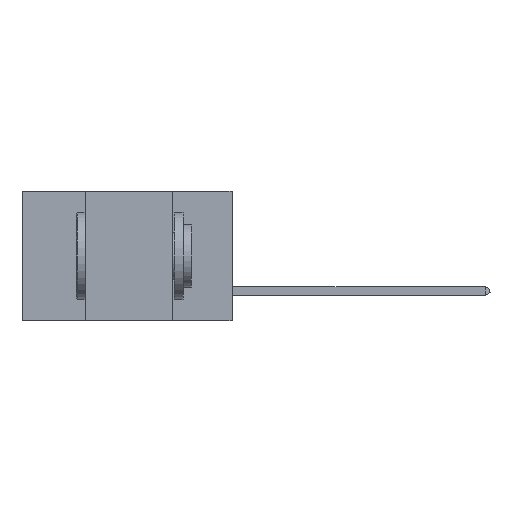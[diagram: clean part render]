
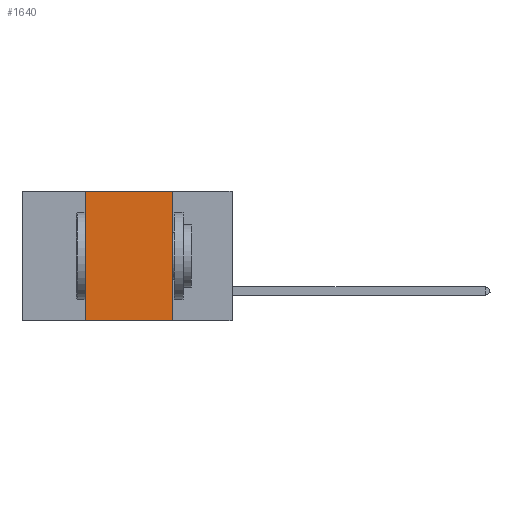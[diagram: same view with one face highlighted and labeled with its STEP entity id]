
A CAD part, left-side view. The second image highlights one B-rep face of the part: STEP entity #1640.
In plain terms, the highlighted planar face has unit normal (-1, 0, 0).
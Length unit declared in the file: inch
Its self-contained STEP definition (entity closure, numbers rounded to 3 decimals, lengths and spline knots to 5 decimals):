
#347 = VERTEX_POINT ( 'NONE', #4210 ) ;
#1179 = DIRECTION ( 'NONE',  ( 0., 0., -1. ) ) ;
#1640 = ADVANCED_FACE ( 'NONE', ( #12622 ), #4724, .F. ) ;
#1885 = CARTESIAN_POINT ( 'NONE',  ( 0., 0.17, 0. ) ) ;
#2037 = VECTOR ( 'NONE', #13070, 39.37008 ) ;
#3229 = VERTEX_POINT ( 'NONE', #1885 ) ;
#3292 = LINE ( 'NONE', #4136, #15643 ) ;
#4108 = EDGE_CURVE ( 'NONE', #347, #5937, #15225, .T. ) ;
#4136 = CARTESIAN_POINT ( 'NONE',  ( 0., 0.6, 0. ) ) ;
#4210 = CARTESIAN_POINT ( 'NONE',  ( 0., 0.42, -0.37 ) ) ;
#4724 = PLANE ( 'NONE',  #19978 ) ;
#4858 = DIRECTION ( 'NONE',  ( 1., 0., 0. ) ) ;
#4985 = LINE ( 'NONE', #20111, #16313 ) ;
#5413 = CARTESIAN_POINT ( 'NONE',  ( 0., 0.42, 0. ) ) ;
#5586 = VECTOR ( 'NONE', #18313, 39.37008 ) ;
#5937 = VERTEX_POINT ( 'NONE', #5413 ) ;
#6559 = ORIENTED_EDGE ( 'NONE', *, *, #7657, .F. ) ;
#7657 = EDGE_CURVE ( 'NONE', #5937, #3229, #3292, .T. ) ;
#7840 = CARTESIAN_POINT ( 'NONE',  ( 0., 0.6, 0. ) ) ;
#8674 = EDGE_CURVE ( 'NONE', #3229, #16984, #4985, .T. ) ;
#10246 = DIRECTION ( 'NONE',  ( 0., -1., 0. ) ) ;
#10285 = CARTESIAN_POINT ( 'NONE',  ( 0., 0.17, -0.37 ) ) ;
#10516 = ORIENTED_EDGE ( 'NONE', *, *, #18574, .T. ) ;
#12622 = FACE_OUTER_BOUND ( 'NONE', #14858, .T. ) ;
#13070 = DIRECTION ( 'NONE',  ( 0., -1., 0. ) ) ;
#14394 = DIRECTION ( 'NONE',  ( 0., 0., -1. ) ) ;
#14858 = EDGE_LOOP ( 'NONE', ( #19906, #6559, #18396, #10516 ) ) ;
#14912 = CARTESIAN_POINT ( 'NONE',  ( 0., 0.6, -0.37 ) ) ;
#15225 = LINE ( 'NONE', #16686, #5586 ) ;
#15643 = VECTOR ( 'NONE', #10246, 39.37008 ) ;
#16313 = VECTOR ( 'NONE', #1179, 39.37008 ) ;
#16686 = CARTESIAN_POINT ( 'NONE',  ( 0., 0.42, 0. ) ) ;
#16836 = LINE ( 'NONE', #14912, #2037 ) ;
#16984 = VERTEX_POINT ( 'NONE', #10285 ) ;
#18313 = DIRECTION ( 'NONE',  ( 0., 0., 1. ) ) ;
#18396 = ORIENTED_EDGE ( 'NONE', *, *, #4108, .F. ) ;
#18574 = EDGE_CURVE ( 'NONE', #347, #16984, #16836, .T. ) ;
#19906 = ORIENTED_EDGE ( 'NONE', *, *, #8674, .F. ) ;
#19978 = AXIS2_PLACEMENT_3D ( 'NONE', #7840, #4858, #14394 ) ;
#20111 = CARTESIAN_POINT ( 'NONE',  ( 0., 0.17, 0. ) ) ;
